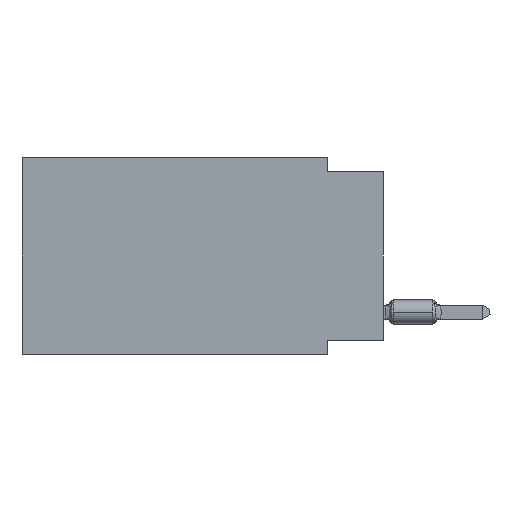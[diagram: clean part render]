
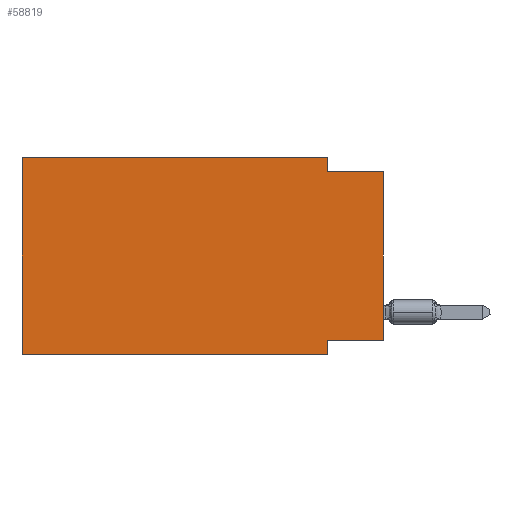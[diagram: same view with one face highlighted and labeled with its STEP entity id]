
A CAD part, left-side view. The second image highlights one B-rep face of the part: STEP entity #58819.
In plain terms, the highlighted planar face has unit normal (-1, 0, 0).
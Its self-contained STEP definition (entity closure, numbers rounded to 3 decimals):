
#86 = VERTEX_POINT ( 'NONE', #8453 ) ;
#124 = CARTESIAN_POINT ( 'NONE',  ( 0., 16.383, 0. ) ) ;
#588 = DIRECTION ( 'NONE',  ( 0., 0., -1. ) ) ;
#712 = EDGE_CURVE ( 'NONE', #80371, #86, #66518, .T. ) ;
#1293 = ORIENTED_EDGE ( 'NONE', *, *, #67960, .F. ) ;
#5221 = LINE ( 'NONE', #67975, #86166 ) ;
#8453 = CARTESIAN_POINT ( 'NONE',  ( 0., 0., -0.635 ) ) ;
#8718 = LINE ( 'NONE', #23372, #9132 ) ;
#9058 = ORIENTED_EDGE ( 'NONE', *, *, #34716, .T. ) ;
#9132 = VECTOR ( 'NONE', #85683, 1000. ) ;
#10380 = VECTOR ( 'NONE', #69644, 1000. ) ;
#10449 = CARTESIAN_POINT ( 'NONE',  ( 0., 16.383, 0. ) ) ;
#12470 = VERTEX_POINT ( 'NONE', #44757 ) ;
#12873 = ORIENTED_EDGE ( 'NONE', *, *, #18927, .F. ) ;
#14318 = EDGE_CURVE ( 'NONE', #71801, #45963, #5221, .T. ) ;
#14815 = ORIENTED_EDGE ( 'NONE', *, *, #88953, .F. ) ;
#15117 = VERTEX_POINT ( 'NONE', #16936 ) ;
#16936 = CARTESIAN_POINT ( 'NONE',  ( 0., 2.54, 0. ) ) ;
#18927 = EDGE_CURVE ( 'NONE', #15117, #80371, #52232, .T. ) ;
#19062 = VERTEX_POINT ( 'NONE', #85756 ) ;
#19606 = ORIENTED_EDGE ( 'NONE', *, *, #86357, .F. ) ;
#20590 = DIRECTION ( 'NONE',  ( 0., 0., 1. ) ) ;
#21098 = VECTOR ( 'NONE', #65376, 1000. ) ;
#21260 = DIRECTION ( 'NONE',  ( 0., 0., -1. ) ) ;
#23372 = CARTESIAN_POINT ( 'NONE',  ( 0., 16.383, 0. ) ) ;
#25828 = DIRECTION ( 'NONE',  ( 0., 1., 0. ) ) ;
#26573 = LINE ( 'NONE', #76933, #48759 ) ;
#28063 = DIRECTION ( 'NONE',  ( 1., 0., 0. ) ) ;
#28167 = VECTOR ( 'NONE', #66420, 1000. ) ;
#28238 = ORIENTED_EDGE ( 'NONE', *, *, #14318, .F. ) ;
#29483 = CARTESIAN_POINT ( 'NONE',  ( 0., 2.54, -0.635 ) ) ;
#31170 = EDGE_LOOP ( 'NONE', ( #9058, #60300, #12873, #1293, #14815, #43088, #19606, #28238 ) ) ;
#34716 = EDGE_CURVE ( 'NONE', #71801, #86, #26573, .T. ) ;
#34843 = CARTESIAN_POINT ( 'NONE',  ( 0., 0., -0.635 ) ) ;
#35380 = FACE_OUTER_BOUND ( 'NONE', #31170, .T. ) ;
#36359 = LINE ( 'NONE', #83561, #57233 ) ;
#37612 = CARTESIAN_POINT ( 'NONE',  ( 0., 2.54, -8.255 ) ) ;
#42142 = AXIS2_PLACEMENT_3D ( 'NONE', #124, #28063, #588 ) ;
#43088 = ORIENTED_EDGE ( 'NONE', *, *, #69610, .T. ) ;
#44757 = CARTESIAN_POINT ( 'NONE',  ( 0., 16.383, -8.89 ) ) ;
#45963 = VERTEX_POINT ( 'NONE', #37612 ) ;
#48759 = VECTOR ( 'NONE', #20590, 1000. ) ;
#52232 = LINE ( 'NONE', #81054, #28167 ) ;
#54368 = VECTOR ( 'NONE', #74036, 1000. ) ;
#57233 = VECTOR ( 'NONE', #21260, 1000. ) ;
#58775 = CARTESIAN_POINT ( 'NONE',  ( 0., 0., -8.255 ) ) ;
#58819 = ADVANCED_FACE ( 'NONE', ( #35380 ), #63323, .F. ) ;
#60300 = ORIENTED_EDGE ( 'NONE', *, *, #712, .F. ) ;
#61933 = VERTEX_POINT ( 'NONE', #10449 ) ;
#63323 = PLANE ( 'NONE',  #42142 ) ;
#63569 = LINE ( 'NONE', #64475, #21098 ) ;
#64475 = CARTESIAN_POINT ( 'NONE',  ( 0., 16.383, -8.89 ) ) ;
#65376 = DIRECTION ( 'NONE',  ( 0., -1., 0. ) ) ;
#66420 = DIRECTION ( 'NONE',  ( 0., 0., -1. ) ) ;
#66518 = LINE ( 'NONE', #34843, #10380 ) ;
#67157 = LINE ( 'NONE', #87316, #54368 ) ;
#67960 = EDGE_CURVE ( 'NONE', #61933, #15117, #8718, .T. ) ;
#67975 = CARTESIAN_POINT ( 'NONE',  ( 0., 0., -8.255 ) ) ;
#69610 = EDGE_CURVE ( 'NONE', #12470, #19062, #63569, .T. ) ;
#69644 = DIRECTION ( 'NONE',  ( 0., -1., 0. ) ) ;
#71801 = VERTEX_POINT ( 'NONE', #58775 ) ;
#74036 = DIRECTION ( 'NONE',  ( 0., 0., 1. ) ) ;
#76933 = CARTESIAN_POINT ( 'NONE',  ( 0., 0., 0. ) ) ;
#80371 = VERTEX_POINT ( 'NONE', #29483 ) ;
#81054 = CARTESIAN_POINT ( 'NONE',  ( 0., 2.54, 0. ) ) ;
#83561 = CARTESIAN_POINT ( 'NONE',  ( 0., 2.54, -8.89 ) ) ;
#85683 = DIRECTION ( 'NONE',  ( 0., -1., 0. ) ) ;
#85756 = CARTESIAN_POINT ( 'NONE',  ( 0., 2.54, -8.89 ) ) ;
#86166 = VECTOR ( 'NONE', #25828, 1000. ) ;
#86357 = EDGE_CURVE ( 'NONE', #45963, #19062, #36359, .T. ) ;
#87316 = CARTESIAN_POINT ( 'NONE',  ( 0., 16.383, 0. ) ) ;
#88953 = EDGE_CURVE ( 'NONE', #12470, #61933, #67157, .T. ) ;
